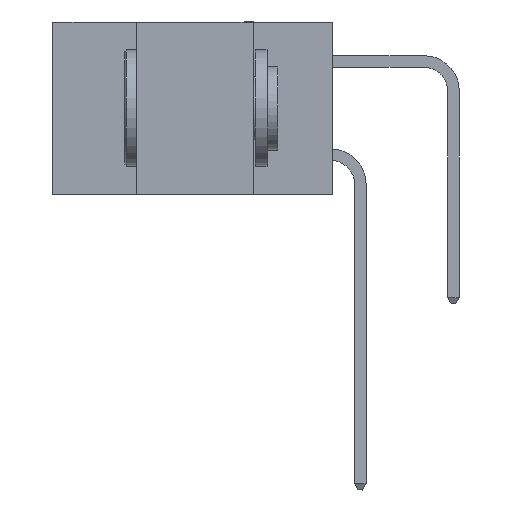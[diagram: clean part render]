
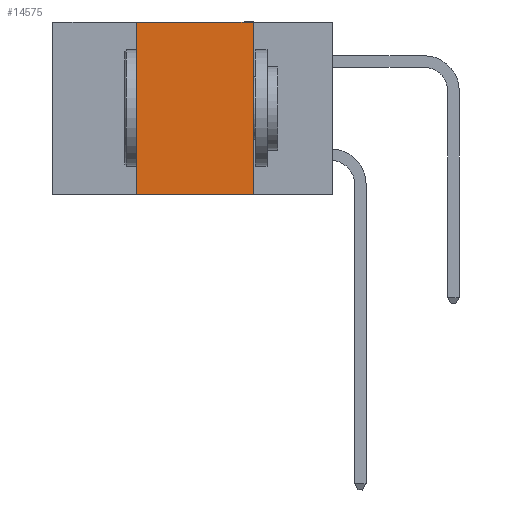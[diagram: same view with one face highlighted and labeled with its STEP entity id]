
A CAD part, left-side view. The second image highlights one B-rep face of the part: STEP entity #14575.
In plain terms, the highlighted planar face has unit normal (-1, 0, 0).
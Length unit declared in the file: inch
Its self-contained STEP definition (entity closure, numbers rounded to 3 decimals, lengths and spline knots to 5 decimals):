
#274 = ORIENTED_EDGE ( 'NONE', *, *, #12007, .F. ) ;
#486 = VECTOR ( 'NONE', #13081, 39.37008 ) ;
#623 = LINE ( 'NONE', #16676, #14900 ) ;
#1273 = AXIS2_PLACEMENT_3D ( 'NONE', #4873, #18951, #6956 ) ;
#1638 = EDGE_CURVE ( 'NONE', #8449, #20474, #11368, .T. ) ;
#1663 = VERTEX_POINT ( 'NONE', #24055 ) ;
#2523 = CARTESIAN_POINT ( 'NONE',  ( 0., 0.6, -0.37 ) ) ;
#2596 = ORIENTED_EDGE ( 'NONE', *, *, #1638, .F. ) ;
#4220 = ORIENTED_EDGE ( 'NONE', *, *, #4331, .F. ) ;
#4331 = EDGE_CURVE ( 'NONE', #10546, #8449, #15361, .T. ) ;
#4873 = CARTESIAN_POINT ( 'NONE',  ( 0., 0.6, 0. ) ) ;
#5608 = CARTESIAN_POINT ( 'NONE',  ( 0., 0.42, -0.37 ) ) ;
#6108 = CARTESIAN_POINT ( 'NONE',  ( 0., 0.42, 0. ) ) ;
#6132 = CARTESIAN_POINT ( 'NONE',  ( 0., 0.17, 0. ) ) ;
#6276 = DIRECTION ( 'NONE',  ( 0., 0., 1. ) ) ;
#6956 = DIRECTION ( 'NONE',  ( 0., 0., -1. ) ) ;
#7393 = CARTESIAN_POINT ( 'NONE',  ( 0., 0.42, 0. ) ) ;
#8449 = VERTEX_POINT ( 'NONE', #7393 ) ;
#8896 = VECTOR ( 'NONE', #14691, 39.37008 ) ;
#9670 = CARTESIAN_POINT ( 'NONE',  ( 0., 0.6, 0. ) ) ;
#10546 = VERTEX_POINT ( 'NONE', #5608 ) ;
#10735 = EDGE_LOOP ( 'NONE', ( #274, #2596, #4220, #21327 ) ) ;
#11368 = LINE ( 'NONE', #9670, #486 ) ;
#12007 = EDGE_CURVE ( 'NONE', #20474, #1663, #623, .T. ) ;
#13081 = DIRECTION ( 'NONE',  ( 0., -1., 0. ) ) ;
#13828 = EDGE_CURVE ( 'NONE', #10546, #1663, #20159, .T. ) ;
#14575 = ADVANCED_FACE ( 'NONE', ( #22583 ), #14910, .F. ) ;
#14691 = DIRECTION ( 'NONE',  ( 0., -1., 0. ) ) ;
#14900 = VECTOR ( 'NONE', #22731, 39.37008 ) ;
#14910 = PLANE ( 'NONE',  #1273 ) ;
#15361 = LINE ( 'NONE', #6108, #20103 ) ;
#16676 = CARTESIAN_POINT ( 'NONE',  ( 0., 0.17, 0. ) ) ;
#18951 = DIRECTION ( 'NONE',  ( 1., 0., 0. ) ) ;
#20103 = VECTOR ( 'NONE', #6276, 39.37008 ) ;
#20159 = LINE ( 'NONE', #2523, #8896 ) ;
#20474 = VERTEX_POINT ( 'NONE', #6132 ) ;
#21327 = ORIENTED_EDGE ( 'NONE', *, *, #13828, .T. ) ;
#22583 = FACE_OUTER_BOUND ( 'NONE', #10735, .T. ) ;
#22731 = DIRECTION ( 'NONE',  ( 0., 0., -1. ) ) ;
#24055 = CARTESIAN_POINT ( 'NONE',  ( 0., 0.17, -0.37 ) ) ;
